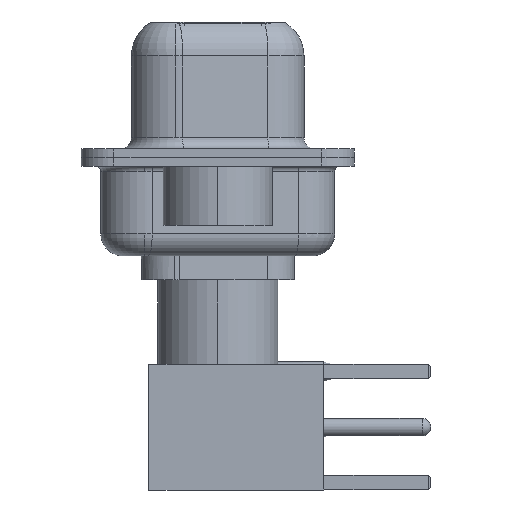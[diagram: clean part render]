
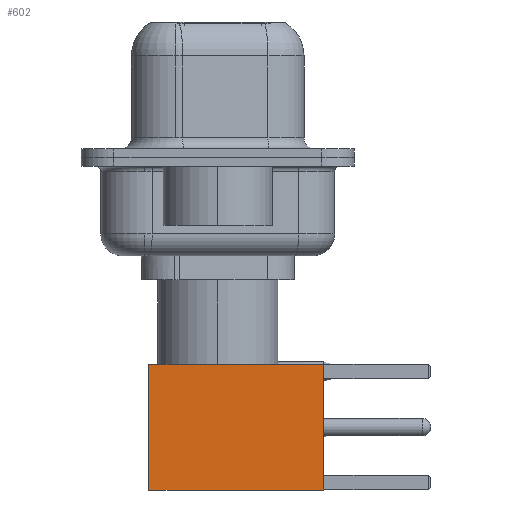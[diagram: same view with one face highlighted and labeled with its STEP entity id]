
A CAD part, left-side view. The second image highlights one B-rep face of the part: STEP entity #602.
In plain terms, the highlighted face is planar.
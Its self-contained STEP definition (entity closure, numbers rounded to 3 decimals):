
#269 = DIRECTION ( 'NONE',  ( 0., 0., -1. ) ) ;
#602 = ADVANCED_FACE ( 'NONE', ( #19616 ), #16501, .T. ) ;
#1267 = CARTESIAN_POINT ( 'NONE',  ( 2.875, 2.875, 0. ) ) ;
#1631 = LINE ( 'NONE', #11052, #17940 ) ;
#2775 = CARTESIAN_POINT ( 'NONE',  ( 2.875, 2.875, 8. ) ) ;
#3059 = LINE ( 'NONE', #3252, #11915 ) ;
#3252 = CARTESIAN_POINT ( 'NONE',  ( -2.875, 2.875, 0. ) ) ;
#3784 = EDGE_CURVE ( 'NONE', #19767, #16549, #1631, .T. ) ;
#4264 = CARTESIAN_POINT ( 'NONE',  ( -2.875, 2.875, 0. ) ) ;
#5051 = EDGE_CURVE ( 'NONE', #18209, #19767, #9251, .T. ) ;
#5185 = EDGE_LOOP ( 'NONE', ( #17833, #5965, #5687, #17310 ) ) ;
#5513 = CARTESIAN_POINT ( 'NONE',  ( 2.875, 2.875, 0. ) ) ;
#5687 = ORIENTED_EDGE ( 'NONE', *, *, #11444, .F. ) ;
#5965 = ORIENTED_EDGE ( 'NONE', *, *, #3784, .T. ) ;
#9251 = LINE ( 'NONE', #1267, #15454 ) ;
#9780 = CARTESIAN_POINT ( 'NONE',  ( 2.875, 2.875, 0. ) ) ;
#10543 = AXIS2_PLACEMENT_3D ( 'NONE', #5513, #11764, #18059 ) ;
#11047 = LINE ( 'NONE', #11356, #11705 ) ;
#11052 = CARTESIAN_POINT ( 'NONE',  ( 0., 2.875, 0. ) ) ;
#11356 = CARTESIAN_POINT ( 'NONE',  ( 0., 2.875, 8. ) ) ;
#11444 = EDGE_CURVE ( 'NONE', #19173, #16549, #3059, .T. ) ;
#11705 = VECTOR ( 'NONE', #17330, 1000. ) ;
#11764 = DIRECTION ( 'NONE',  ( 0., 1., 0. ) ) ;
#11915 = VECTOR ( 'NONE', #269, 1000. ) ;
#15454 = VECTOR ( 'NONE', #18409, 1000. ) ;
#16160 = EDGE_CURVE ( 'NONE', #18209, #19173, #11047, .T. ) ;
#16501 = PLANE ( 'NONE',  #10543 ) ;
#16549 = VERTEX_POINT ( 'NONE', #4264 ) ;
#17130 = DIRECTION ( 'NONE',  ( -1., 0., 0. ) ) ;
#17310 = ORIENTED_EDGE ( 'NONE', *, *, #16160, .F. ) ;
#17330 = DIRECTION ( 'NONE',  ( -1., 0., 0. ) ) ;
#17833 = ORIENTED_EDGE ( 'NONE', *, *, #5051, .T. ) ;
#17940 = VECTOR ( 'NONE', #17130, 1000. ) ;
#18059 = DIRECTION ( 'NONE',  ( 0., 0., 1. ) ) ;
#18209 = VERTEX_POINT ( 'NONE', #2775 ) ;
#18409 = DIRECTION ( 'NONE',  ( 0., 0., -1. ) ) ;
#19173 = VERTEX_POINT ( 'NONE', #20312 ) ;
#19616 = FACE_OUTER_BOUND ( 'NONE', #5185, .T. ) ;
#19767 = VERTEX_POINT ( 'NONE', #9780 ) ;
#20312 = CARTESIAN_POINT ( 'NONE',  ( -2.875, 2.875, 8. ) ) ;
